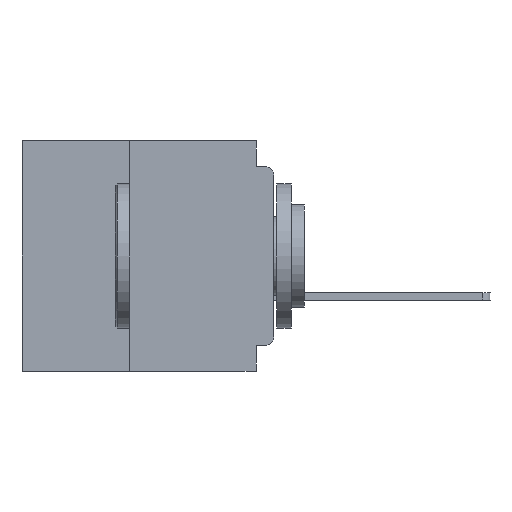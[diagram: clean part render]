
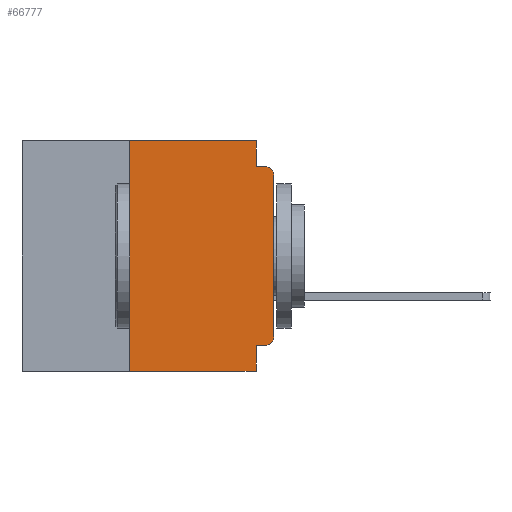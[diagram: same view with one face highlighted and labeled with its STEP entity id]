
A CAD part, left-side view. The second image highlights one B-rep face of the part: STEP entity #66777.
In plain terms, the highlighted planar face has unit normal (-1, 0, 0).
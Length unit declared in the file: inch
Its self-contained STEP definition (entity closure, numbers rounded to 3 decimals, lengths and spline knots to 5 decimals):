
#565 = VERTEX_POINT ( 'NONE', #7908 ) ;
#949 = EDGE_CURVE ( 'NONE', #44295, #5260, #59716, .T. ) ;
#2003 = VECTOR ( 'NONE', #61126, 39.37008 ) ;
#2256 = PLANE ( 'NONE',  #43826 ) ;
#2366 = ORIENTED_EDGE ( 'NONE', *, *, #31641, .F. ) ;
#2991 = EDGE_CURVE ( 'NONE', #33201, #565, #23506, .T. ) ;
#4001 = AXIS2_PLACEMENT_3D ( 'NONE', #48939, #16854, #54314 ) ;
#4096 = LINE ( 'NONE', #12127, #57718 ) ;
#5260 = VERTEX_POINT ( 'NONE', #18565 ) ;
#5959 = DIRECTION ( 'NONE',  ( 0., 0., 1. ) ) ;
#6302 = ORIENTED_EDGE ( 'NONE', *, *, #949, .F. ) ;
#7372 = DIRECTION ( 'NONE',  ( 0., 0., -1. ) ) ;
#7908 = CARTESIAN_POINT ( 'NONE',  ( 0., 0.25, 0. ) ) ;
#8353 = EDGE_CURVE ( 'NONE', #23619, #29027, #64093, .T. ) ;
#10247 = DIRECTION ( 'NONE',  ( 0., 1., 0. ) ) ;
#12127 = CARTESIAN_POINT ( 'NONE',  ( 0., 0., 0. ) ) ;
#12899 = LINE ( 'NONE', #29418, #2003 ) ;
#15038 = ORIENTED_EDGE ( 'NONE', *, *, #2991, .F. ) ;
#16233 = CARTESIAN_POINT ( 'NONE',  ( 0., 0.437, -0.4 ) ) ;
#16854 = DIRECTION ( 'NONE',  ( -1., 0., 0. ) ) ;
#17384 = DIRECTION ( 'NONE',  ( 0., -1., 0. ) ) ;
#17908 = VECTOR ( 'NONE', #7372, 39.37008 ) ;
#18565 = CARTESIAN_POINT ( 'NONE',  ( 0., 0.031, -0.4 ) ) ;
#19384 = EDGE_LOOP ( 'NONE', ( #24702, #32894, #22300, #2366, #40448, #15038, #52567, #6302, #52007, #43141 ) ) ;
#19655 = DIRECTION ( 'NONE',  ( -1., 0., 0. ) ) ;
#20110 = CIRCLE ( 'NONE', #4001, 0.015 ) ;
#20394 = EDGE_CURVE ( 'NONE', #23619, #44295, #24355, .T. ) ;
#21551 = CARTESIAN_POINT ( 'NONE',  ( 0., 0., -0.34 ) ) ;
#21678 = DIRECTION ( 'NONE',  ( 0., -1., 0. ) ) ;
#22300 = ORIENTED_EDGE ( 'NONE', *, *, #60219, .F. ) ;
#23388 = CARTESIAN_POINT ( 'NONE',  ( 0., 0.031, 0. ) ) ;
#23506 = LINE ( 'NONE', #53978, #50235 ) ;
#23619 = VERTEX_POINT ( 'NONE', #44426 ) ;
#23942 = DIRECTION ( 'NONE',  ( 1., 0., 0. ) ) ;
#24355 = LINE ( 'NONE', #47754, #38504 ) ;
#24702 = ORIENTED_EDGE ( 'NONE', *, *, #39372, .T. ) ;
#25799 = LINE ( 'NONE', #28236, #27491 ) ;
#26873 = CARTESIAN_POINT ( 'NONE',  ( 0., 0.031, 0. ) ) ;
#27491 = VECTOR ( 'NONE', #17384, 39.37008 ) ;
#28236 = CARTESIAN_POINT ( 'NONE',  ( 0., 0., -0.045 ) ) ;
#28412 = DIRECTION ( 'NONE',  ( 0., 0., 1. ) ) ;
#29027 = VERTEX_POINT ( 'NONE', #21551 ) ;
#29418 = CARTESIAN_POINT ( 'NONE',  ( 0., 0.437, 0. ) ) ;
#29689 = VECTOR ( 'NONE', #59951, 39.37008 ) ;
#31641 = EDGE_CURVE ( 'NONE', #46467, #50553, #32215, .T. ) ;
#32215 = LINE ( 'NONE', #23388, #17908 ) ;
#32894 = ORIENTED_EDGE ( 'NONE', *, *, #58886, .T. ) ;
#33201 = VERTEX_POINT ( 'NONE', #66383 ) ;
#34450 = CARTESIAN_POINT ( 'NONE',  ( 0., 0.437, 0. ) ) ;
#37816 = CARTESIAN_POINT ( 'NONE',  ( 0., 0.031, -0.045 ) ) ;
#38504 = VECTOR ( 'NONE', #10247, 39.37008 ) ;
#39372 = EDGE_CURVE ( 'NONE', #29027, #60738, #4096, .T. ) ;
#40448 = ORIENTED_EDGE ( 'NONE', *, *, #52507, .F. ) ;
#40458 = EDGE_CURVE ( 'NONE', #33201, #5260, #41506, .T. ) ;
#41506 = LINE ( 'NONE', #16233, #68197 ) ;
#43141 = ORIENTED_EDGE ( 'NONE', *, *, #8353, .T. ) ;
#43826 = AXIS2_PLACEMENT_3D ( 'NONE', #34450, #23942, #61245 ) ;
#44295 = VERTEX_POINT ( 'NONE', #46920 ) ;
#44426 = CARTESIAN_POINT ( 'NONE',  ( 0., 0.015, -0.355 ) ) ;
#46467 = VERTEX_POINT ( 'NONE', #26873 ) ;
#46920 = CARTESIAN_POINT ( 'NONE',  ( 0., 0.031, -0.355 ) ) ;
#47754 = CARTESIAN_POINT ( 'NONE',  ( 0., 0., -0.355 ) ) ;
#48939 = CARTESIAN_POINT ( 'NONE',  ( 0., 0.015, -0.06 ) ) ;
#50235 = VECTOR ( 'NONE', #5959, 39.37008 ) ;
#50553 = VERTEX_POINT ( 'NONE', #37816 ) ;
#51113 = AXIS2_PLACEMENT_3D ( 'NONE', #51706, #19655, #57088 ) ;
#51706 = CARTESIAN_POINT ( 'NONE',  ( 0., 0.015, -0.34 ) ) ;
#52007 = ORIENTED_EDGE ( 'NONE', *, *, #20394, .F. ) ;
#52507 = EDGE_CURVE ( 'NONE', #565, #46467, #12899, .T. ) ;
#52567 = ORIENTED_EDGE ( 'NONE', *, *, #40458, .T. ) ;
#53978 = CARTESIAN_POINT ( 'NONE',  ( 0., 0.25, -0.4 ) ) ;
#54012 = VERTEX_POINT ( 'NONE', #69190 ) ;
#54314 = DIRECTION ( 'NONE',  ( 0., 0., -1. ) ) ;
#57088 = DIRECTION ( 'NONE',  ( 0., 0., -1. ) ) ;
#57718 = VECTOR ( 'NONE', #28412, 39.37008 ) ;
#58886 = EDGE_CURVE ( 'NONE', #60738, #54012, #20110, .T. ) ;
#59413 = CARTESIAN_POINT ( 'NONE',  ( 0., 0., -0.06 ) ) ;
#59716 = LINE ( 'NONE', #60625, #29689 ) ;
#59951 = DIRECTION ( 'NONE',  ( 0., 0., -1. ) ) ;
#60070 = FACE_OUTER_BOUND ( 'NONE', #19384, .T. ) ;
#60219 = EDGE_CURVE ( 'NONE', #50553, #54012, #25799, .T. ) ;
#60625 = CARTESIAN_POINT ( 'NONE',  ( 0., 0.031, -0.4 ) ) ;
#60738 = VERTEX_POINT ( 'NONE', #59413 ) ;
#61126 = DIRECTION ( 'NONE',  ( 0., -1., 0. ) ) ;
#61245 = DIRECTION ( 'NONE',  ( 0., 0., -1. ) ) ;
#64093 = CIRCLE ( 'NONE', #51113, 0.015 ) ;
#66383 = CARTESIAN_POINT ( 'NONE',  ( 0., 0.25, -0.4 ) ) ;
#66777 = ADVANCED_FACE ( 'NONE', ( #60070 ), #2256, .F. ) ;
#68197 = VECTOR ( 'NONE', #21678, 39.37008 ) ;
#69190 = CARTESIAN_POINT ( 'NONE',  ( 0., 0.015, -0.045 ) ) ;
